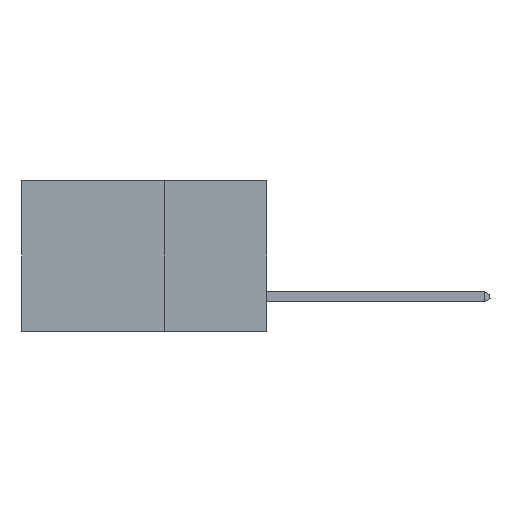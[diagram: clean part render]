
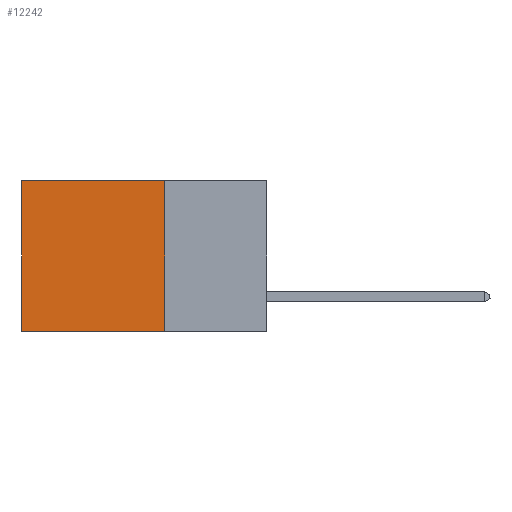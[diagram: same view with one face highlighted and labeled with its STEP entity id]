
A CAD part, left-side view. The second image highlights one B-rep face of the part: STEP entity #12242.
In plain terms, the highlighted planar face has unit normal (-1, 0, 0).
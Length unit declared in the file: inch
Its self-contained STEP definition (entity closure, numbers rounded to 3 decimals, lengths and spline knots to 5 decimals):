
#129 = EDGE_CURVE ( 'NONE', #12617, #12876, #5941, .T. ) ;
#572 = ORIENTED_EDGE ( 'NONE', *, *, #11689, .T. ) ;
#582 = LINE ( 'NONE', #13114, #12286 ) ;
#1908 = DIRECTION ( 'NONE',  ( 0., 0., -1. ) ) ;
#2617 = CARTESIAN_POINT ( 'NONE',  ( 0.2875, 0.25, -0.37 ) ) ;
#2745 = DIRECTION ( 'NONE',  ( 0., 1., 0. ) ) ;
#2962 = LINE ( 'NONE', #5761, #16385 ) ;
#4361 = EDGE_LOOP ( 'NONE', ( #572, #8995, #16423, #5247 ) ) ;
#4598 = DIRECTION ( 'NONE',  ( 1., 0., 0. ) ) ;
#5247 = ORIENTED_EDGE ( 'NONE', *, *, #10154, .T. ) ;
#5761 = CARTESIAN_POINT ( 'NONE',  ( 0.2875, 0.25, 0. ) ) ;
#5903 = CARTESIAN_POINT ( 'NONE',  ( 0.2875, 0.6, -0.37 ) ) ;
#5941 = LINE ( 'NONE', #6592, #8638 ) ;
#5951 = CARTESIAN_POINT ( 'NONE',  ( 0.2875, 0.6, 0. ) ) ;
#6592 = CARTESIAN_POINT ( 'NONE',  ( 0.2875, 0.25, 0. ) ) ;
#7018 = DIRECTION ( 'NONE',  ( 0., 1., 0. ) ) ;
#7319 = PLANE ( 'NONE',  #10768 ) ;
#7409 = VECTOR ( 'NONE', #2745, 39.37008 ) ;
#7858 = DIRECTION ( 'NONE',  ( 0., 0., -1. ) ) ;
#8638 = VECTOR ( 'NONE', #11822, 39.37008 ) ;
#8738 = EDGE_CURVE ( 'NONE', #12876, #11682, #13908, .T. ) ;
#8995 = ORIENTED_EDGE ( 'NONE', *, *, #8738, .F. ) ;
#9744 = FACE_OUTER_BOUND ( 'NONE', #4361, .T. ) ;
#10154 = EDGE_CURVE ( 'NONE', #12617, #14196, #2962, .T. ) ;
#10571 = CARTESIAN_POINT ( 'NONE',  ( 0.2875, 0.25, -0.37 ) ) ;
#10768 = AXIS2_PLACEMENT_3D ( 'NONE', #13982, #4598, #1908 ) ;
#11682 = VERTEX_POINT ( 'NONE', #5903 ) ;
#11689 = EDGE_CURVE ( 'NONE', #14196, #11682, #582, .T. ) ;
#11822 = DIRECTION ( 'NONE',  ( 0., 0., -1. ) ) ;
#12242 = ADVANCED_FACE ( 'NONE', ( #9744 ), #7319, .F. ) ;
#12286 = VECTOR ( 'NONE', #7858, 39.37008 ) ;
#12617 = VERTEX_POINT ( 'NONE', #15018 ) ;
#12876 = VERTEX_POINT ( 'NONE', #2617 ) ;
#13114 = CARTESIAN_POINT ( 'NONE',  ( 0.2875, 0.6, 0. ) ) ;
#13908 = LINE ( 'NONE', #10571, #7409 ) ;
#13982 = CARTESIAN_POINT ( 'NONE',  ( 0.2875, 0.25, 0. ) ) ;
#14196 = VERTEX_POINT ( 'NONE', #5951 ) ;
#15018 = CARTESIAN_POINT ( 'NONE',  ( 0.2875, 0.25, 0. ) ) ;
#16385 = VECTOR ( 'NONE', #7018, 39.37008 ) ;
#16423 = ORIENTED_EDGE ( 'NONE', *, *, #129, .F. ) ;
